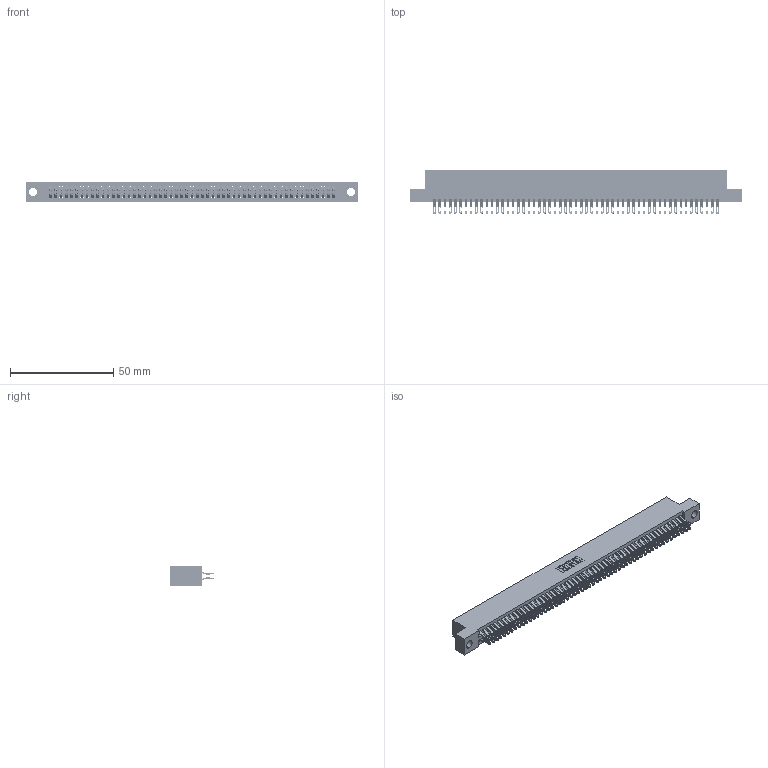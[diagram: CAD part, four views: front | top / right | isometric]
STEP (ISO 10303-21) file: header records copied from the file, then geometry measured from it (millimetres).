
FILE_DESCRIPTION (( 'STEP AP203' ), '1' );
FILE_NAME ('395-110-555-204.STEP', '2018-12-01T04:26:36', ( '' ), ( '' ), 'SwSTEP 2.0', 'SolidWorks 2016', '' );
FILE_SCHEMA (( 'CONFIG_CONTROL_DESIGN' ));
Length unit declared in the file: inch
Products named in the file (3): 345 Part_Flush Mounting Lugs - 0.156 Dia-TH; 395-110-555-204; 345-292-001_555 Tail
Assembly tree (111 placements, depth 2):
  395-110-555-204
    345 Part_Flush Mounting Lugs - 0.156 Dia-TH
    345-292-001_555 Tail  x110
Bounding box: 160.91 x 21.13 x 9.4 mm (x, y, z)
Volume: 15982.7 mm3; surface area: 24801.9 mm2
Topology: 111 solids, 111 shells, 6286 faces, 19811 edges, 13206 vertices
Faces by surface type: plane 3490, cylinder 2796
Entity records: 41733 total; most frequent: CARTESIAN_POINT 7018, ORIENTED_EDGE 6922, DIRECTION 6141, EDGE_CURVE 3461, LINE 3089, VECTOR 3089, VERTEX_POINT 2306, AXIS2_PLACEMENT_3D 1526
